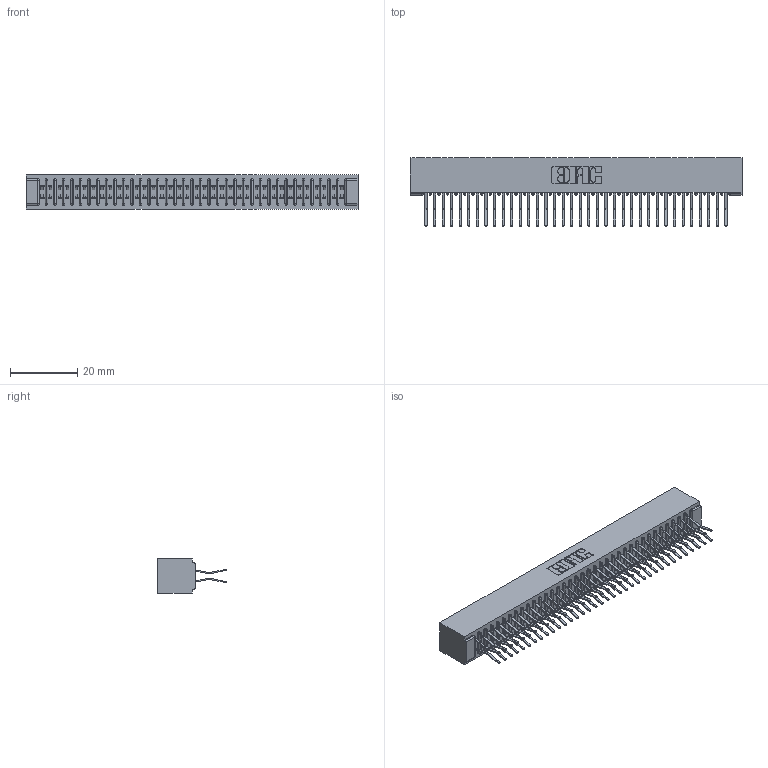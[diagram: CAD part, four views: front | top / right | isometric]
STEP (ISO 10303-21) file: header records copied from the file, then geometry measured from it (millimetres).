
FILE_DESCRIPTION (( 'STEP AP203' ), '1' );
FILE_NAME ('391-072-560-201.STEP', '2018-08-09T14:30:46', ( '' ), ( '' ), 'SwSTEP 2.0', 'SolidWorks 2016', '' );
FILE_SCHEMA (( 'CONFIG_CONTROL_DESIGN' ));
Length unit declared in the file: inch
Products named in the file (3): 341 Part_No Mounting Lugs; 341-292-001_341-292-160; 391-072-560-201
Assembly tree (73 placements, depth 2):
  391-072-560-201
    341 Part_No Mounting Lugs
    341-292-001_341-292-160  x72
Bounding box: 98.42 x 20.37 x 10.16 mm (x, y, z)
Volume: 7570.2 mm3; surface area: 14443.9 mm2
Topology: 73 solids, 73 shells, 5148 faces, 14944 edges, 9694 vertices
Faces by surface type: plane 2944, cylinder 2060, sphere 74, torus 70
Entity records: 44229 total; most frequent: CARTESIAN_POINT 7352, ORIENTED_EDGE 7304, DIRECTION 7142, EDGE_CURVE 3652, VECTOR 2942, LINE 2942, VERTEX_POINT 2310, AXIS2_PLACEMENT_3D 2100
